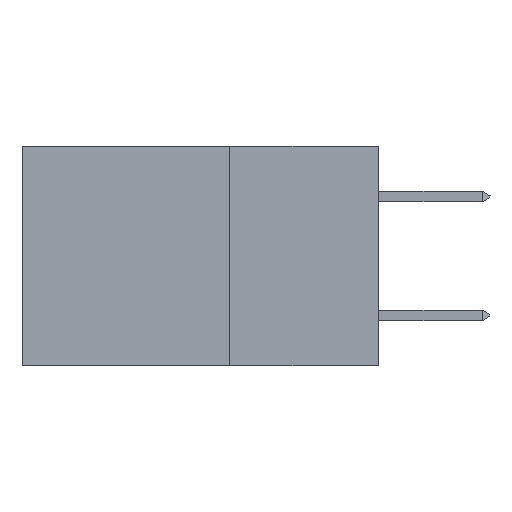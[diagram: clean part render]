
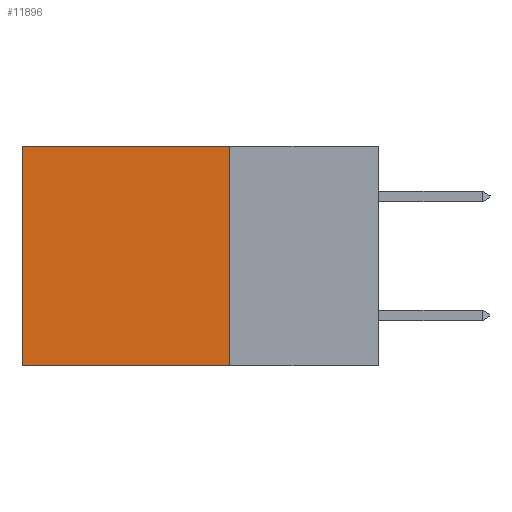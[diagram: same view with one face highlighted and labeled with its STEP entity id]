
A CAD part, left-side view. The second image highlights one B-rep face of the part: STEP entity #11896.
In plain terms, the highlighted planar face has unit normal (-1, 0, 0).
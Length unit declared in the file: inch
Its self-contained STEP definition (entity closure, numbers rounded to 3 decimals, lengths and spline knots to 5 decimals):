
#705 = CARTESIAN_POINT ( 'NONE',  ( 0.2615, 0.6, -0.37 ) ) ;
#1273 = ORIENTED_EDGE ( 'NONE', *, *, #7544, .F. ) ;
#1639 = EDGE_CURVE ( 'NONE', #4562, #4850, #5801, .T. ) ;
#1707 = FACE_OUTER_BOUND ( 'NONE', #9024, .T. ) ;
#1946 = VERTEX_POINT ( 'NONE', #11889 ) ;
#2055 = DIRECTION ( 'NONE',  ( 0., 1., 0. ) ) ;
#2121 = VERTEX_POINT ( 'NONE', #4593 ) ;
#2795 = VECTOR ( 'NONE', #11007, 39.37008 ) ;
#3809 = ORIENTED_EDGE ( 'NONE', *, *, #12279, .F. ) ;
#4356 = DIRECTION ( 'NONE',  ( 0., 0., -1. ) ) ;
#4562 = VERTEX_POINT ( 'NONE', #12086 ) ;
#4593 = CARTESIAN_POINT ( 'NONE',  ( 0.2615, 0.6, -0.37 ) ) ;
#4651 = CARTESIAN_POINT ( 'NONE',  ( 0.2615, 0.25, 0. ) ) ;
#4850 = VERTEX_POINT ( 'NONE', #6295 ) ;
#5801 = LINE ( 'NONE', #4651, #11310 ) ;
#6012 = DIRECTION ( 'NONE',  ( 1., 0., 0. ) ) ;
#6295 = CARTESIAN_POINT ( 'NONE',  ( 0.2615, 0.6, 0. ) ) ;
#6954 = DIRECTION ( 'NONE',  ( 0., 0., -1. ) ) ;
#7167 = CARTESIAN_POINT ( 'NONE',  ( 0.2615, 0.25, -0.37 ) ) ;
#7247 = VECTOR ( 'NONE', #2055, 39.37008 ) ;
#7544 = EDGE_CURVE ( 'NONE', #4562, #1946, #9460, .T. ) ;
#7741 = VECTOR ( 'NONE', #4356, 39.37008 ) ;
#8235 = AXIS2_PLACEMENT_3D ( 'NONE', #13219, #6012, #6954 ) ;
#8514 = EDGE_CURVE ( 'NONE', #4850, #2121, #12891, .T. ) ;
#8523 = CARTESIAN_POINT ( 'NONE',  ( 0.2615, 0.25, -0.37 ) ) ;
#9024 = EDGE_LOOP ( 'NONE', ( #10916, #3809, #1273, #13073 ) ) ;
#9129 = LINE ( 'NONE', #7167, #7247 ) ;
#9460 = LINE ( 'NONE', #8523, #7741 ) ;
#9896 = DIRECTION ( 'NONE',  ( 0., 1., 0. ) ) ;
#9903 = PLANE ( 'NONE',  #8235 ) ;
#10916 = ORIENTED_EDGE ( 'NONE', *, *, #8514, .T. ) ;
#11007 = DIRECTION ( 'NONE',  ( 0., 0., -1. ) ) ;
#11310 = VECTOR ( 'NONE', #9896, 39.37008 ) ;
#11889 = CARTESIAN_POINT ( 'NONE',  ( 0.2615, 0.25, -0.37 ) ) ;
#11896 = ADVANCED_FACE ( 'NONE', ( #1707 ), #9903, .F. ) ;
#12086 = CARTESIAN_POINT ( 'NONE',  ( 0.2615, 0.25, 0. ) ) ;
#12279 = EDGE_CURVE ( 'NONE', #1946, #2121, #9129, .T. ) ;
#12891 = LINE ( 'NONE', #705, #2795 ) ;
#13073 = ORIENTED_EDGE ( 'NONE', *, *, #1639, .T. ) ;
#13219 = CARTESIAN_POINT ( 'NONE',  ( 0.2615, 0.25, -0.37 ) ) ;
